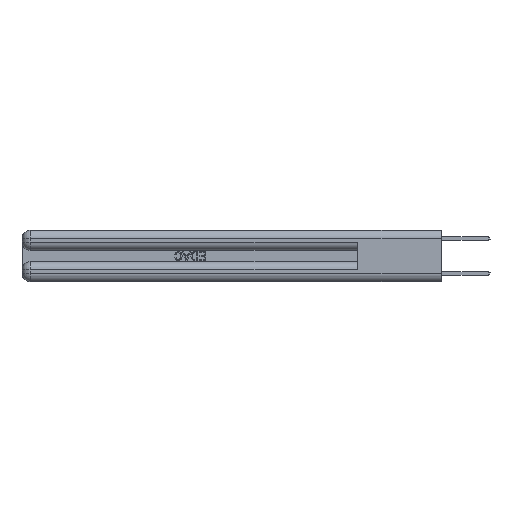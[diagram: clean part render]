
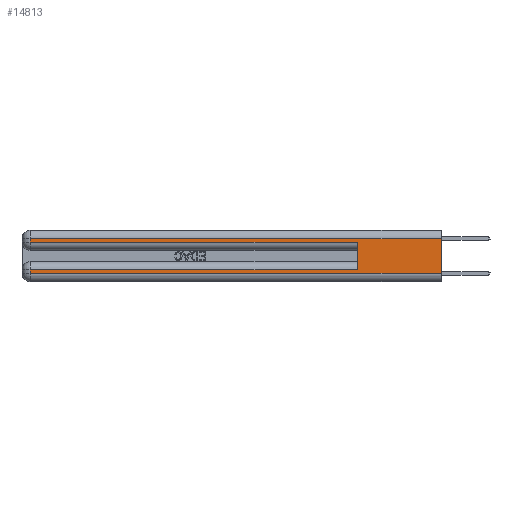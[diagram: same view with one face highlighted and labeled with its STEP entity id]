
A CAD part, left-side view. The second image highlights one B-rep face of the part: STEP entity #14813.
In plain terms, the highlighted planar face has unit normal (-1, 0, 0).
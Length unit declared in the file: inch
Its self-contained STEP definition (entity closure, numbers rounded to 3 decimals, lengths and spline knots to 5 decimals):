
#716 = ORIENTED_EDGE ( 'NONE', *, *, #19775, .T. ) ;
#1194 = EDGE_CURVE ( 'NONE', #20157, #10377, #15165, .T. ) ;
#1195 = ORIENTED_EDGE ( 'NONE', *, *, #1654, .T. ) ;
#1654 = EDGE_CURVE ( 'NONE', #10377, #9403, #30055, .T. ) ;
#1760 = DIRECTION ( 'NONE',  ( 0., 0., 1. ) ) ;
#2397 = VECTOR ( 'NONE', #6744, 39.37008 ) ;
#2978 = ORIENTED_EDGE ( 'NONE', *, *, #22764, .T. ) ;
#3138 = CARTESIAN_POINT ( 'NONE',  ( 0., 0., 0.31 ) ) ;
#3249 = AXIS2_PLACEMENT_3D ( 'NONE', #15290, #23371, #23207 ) ;
#3941 = EDGE_CURVE ( 'NONE', #9661, #20157, #10453, .T. ) ;
#4872 = VECTOR ( 'NONE', #28775, 39.37008 ) ;
#5194 = CARTESIAN_POINT ( 'NONE',  ( 0., 0., 0.37 ) ) ;
#6070 = DIRECTION ( 'NONE',  ( 0., 1., 0. ) ) ;
#6744 = DIRECTION ( 'NONE',  ( 0., -1., 0. ) ) ;
#7621 = DIRECTION ( 'NONE',  ( 0., 0., -1. ) ) ;
#8520 = ORIENTED_EDGE ( 'NONE', *, *, #3941, .T. ) ;
#8649 = EDGE_CURVE ( 'NONE', #10702, #12922, #32446, .T. ) ;
#9403 = VERTEX_POINT ( 'NONE', #13513 ) ;
#9661 = VERTEX_POINT ( 'NONE', #19528 ) ;
#10073 = CARTESIAN_POINT ( 'NONE',  ( 0., 2.94, 0.285 ) ) ;
#10153 = CARTESIAN_POINT ( 'NONE',  ( 0., 2.94, 0.37 ) ) ;
#10377 = VERTEX_POINT ( 'NONE', #15460 ) ;
#10453 = LINE ( 'NONE', #12870, #29329 ) ;
#10702 = VERTEX_POINT ( 'NONE', #10073 ) ;
#11143 = EDGE_CURVE ( 'NONE', #19458, #9403, #20539, .T. ) ;
#11562 = CARTESIAN_POINT ( 'NONE',  ( 0., 0., 0.285 ) ) ;
#12870 = CARTESIAN_POINT ( 'NONE',  ( 0., 0., 0.085 ) ) ;
#12922 = VERTEX_POINT ( 'NONE', #32931 ) ;
#13184 = ORIENTED_EDGE ( 'NONE', *, *, #8649, .T. ) ;
#13488 = LINE ( 'NONE', #3138, #19810 ) ;
#13513 = CARTESIAN_POINT ( 'NONE',  ( 0., 0., 0.06 ) ) ;
#14813 = ADVANCED_FACE ( 'NONE', ( #31003 ), #17374, .F. ) ;
#15165 = LINE ( 'NONE', #10153, #4872 ) ;
#15178 = ORIENTED_EDGE ( 'NONE', *, *, #1194, .T. ) ;
#15290 = CARTESIAN_POINT ( 'NONE',  ( 0., 0., 0.37 ) ) ;
#15460 = CARTESIAN_POINT ( 'NONE',  ( 0., 2.94, 0.06 ) ) ;
#15730 = VERTEX_POINT ( 'NONE', #18413 ) ;
#17374 = PLANE ( 'NONE',  #3249 ) ;
#17383 = DIRECTION ( 'NONE',  ( 0., 0., -1. ) ) ;
#18413 = CARTESIAN_POINT ( 'NONE',  ( 0., 2.94, 0.31 ) ) ;
#19118 = CARTESIAN_POINT ( 'NONE',  ( 0., 2.94, 0.085 ) ) ;
#19458 = VERTEX_POINT ( 'NONE', #28172 ) ;
#19507 = LINE ( 'NONE', #22779, #23665 ) ;
#19528 = CARTESIAN_POINT ( 'NONE',  ( 0., 0.6, 0.085 ) ) ;
#19775 = EDGE_CURVE ( 'NONE', #19458, #15730, #13488, .T. ) ;
#19810 = VECTOR ( 'NONE', #6070, 39.37008 ) ;
#20157 = VERTEX_POINT ( 'NONE', #19118 ) ;
#20463 = LINE ( 'NONE', #33593, #33877 ) ;
#20539 = LINE ( 'NONE', #5194, #27960 ) ;
#21053 = EDGE_CURVE ( 'NONE', #9661, #12922, #19507, .T. ) ;
#22537 = VECTOR ( 'NONE', #29072, 39.37008 ) ;
#22764 = EDGE_CURVE ( 'NONE', #15730, #10702, #20463, .T. ) ;
#22779 = CARTESIAN_POINT ( 'NONE',  ( 0., 0.6, 0.145 ) ) ;
#23207 = DIRECTION ( 'NONE',  ( 0., 0., -1. ) ) ;
#23371 = DIRECTION ( 'NONE',  ( 1., 0., 0. ) ) ;
#23665 = VECTOR ( 'NONE', #1760, 39.37008 ) ;
#23695 = CARTESIAN_POINT ( 'NONE',  ( 0., 0., 0.06 ) ) ;
#25971 = DIRECTION ( 'NONE',  ( 0., 1., 0. ) ) ;
#27960 = VECTOR ( 'NONE', #7621, 39.37008 ) ;
#28172 = CARTESIAN_POINT ( 'NONE',  ( 0., 0., 0.31 ) ) ;
#28775 = DIRECTION ( 'NONE',  ( 0., 0., -1. ) ) ;
#28845 = EDGE_LOOP ( 'NONE', ( #29351, #716, #2978, #13184, #31232, #8520, #15178, #1195 ) ) ;
#29072 = DIRECTION ( 'NONE',  ( 0., -1., 0. ) ) ;
#29329 = VECTOR ( 'NONE', #25971, 39.37008 ) ;
#29351 = ORIENTED_EDGE ( 'NONE', *, *, #11143, .F. ) ;
#30055 = LINE ( 'NONE', #23695, #22537 ) ;
#31003 = FACE_OUTER_BOUND ( 'NONE', #28845, .T. ) ;
#31232 = ORIENTED_EDGE ( 'NONE', *, *, #21053, .F. ) ;
#32446 = LINE ( 'NONE', #11562, #2397 ) ;
#32931 = CARTESIAN_POINT ( 'NONE',  ( 0., 0.6, 0.285 ) ) ;
#33593 = CARTESIAN_POINT ( 'NONE',  ( 0., 2.94, 0.37 ) ) ;
#33877 = VECTOR ( 'NONE', #17383, 39.37008 ) ;
